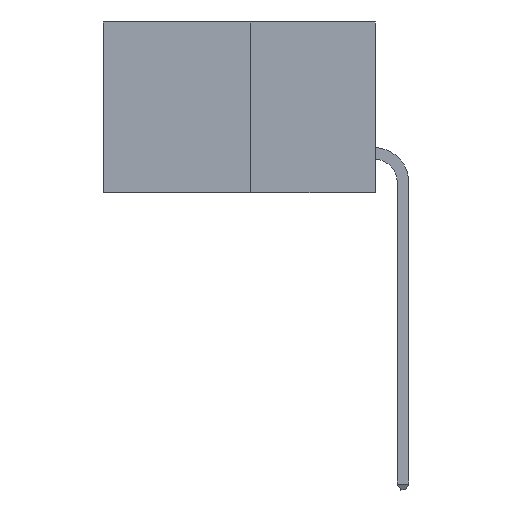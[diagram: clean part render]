
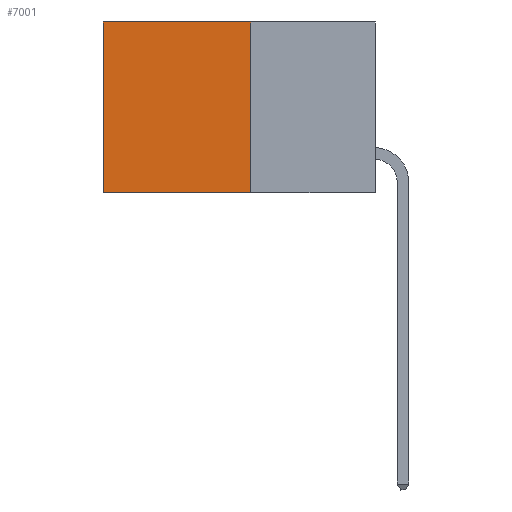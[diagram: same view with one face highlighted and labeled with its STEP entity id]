
A CAD part, left-side view. The second image highlights one B-rep face of the part: STEP entity #7001.
In plain terms, the highlighted planar face has unit normal (-1, 0, 0).
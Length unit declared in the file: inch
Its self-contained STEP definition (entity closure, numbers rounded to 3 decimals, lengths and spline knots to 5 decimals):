
#59 = CARTESIAN_POINT ( 'NONE',  ( 0.277, 0.27, -0.37 ) ) ;
#160 = DIRECTION ( 'NONE',  ( 0., 1., 0. ) ) ;
#420 = VECTOR ( 'NONE', #11114, 39.37008 ) ;
#424 = ORIENTED_EDGE ( 'NONE', *, *, #3359, .T. ) ;
#548 = ORIENTED_EDGE ( 'NONE', *, *, #3813, .T. ) ;
#681 = FACE_OUTER_BOUND ( 'NONE', #6501, .T. ) ;
#788 = LINE ( 'NONE', #7457, #10775 ) ;
#984 = DIRECTION ( 'NONE',  ( 0., 0., -1. ) ) ;
#1108 = LINE ( 'NONE', #9748, #420 ) ;
#2224 = CARTESIAN_POINT ( 'NONE',  ( 0.277, 0.59, -0.37 ) ) ;
#2592 = DIRECTION ( 'NONE',  ( 0., 0., -1. ) ) ;
#3055 = ORIENTED_EDGE ( 'NONE', *, *, #3222, .F. ) ;
#3222 = EDGE_CURVE ( 'NONE', #3779, #10285, #10219, .T. ) ;
#3359 = EDGE_CURVE ( 'NONE', #5537, #12419, #10066, .T. ) ;
#3399 = ORIENTED_EDGE ( 'NONE', *, *, #9076, .F. ) ;
#3779 = VERTEX_POINT ( 'NONE', #4586 ) ;
#3813 = EDGE_CURVE ( 'NONE', #12419, #10285, #1108, .T. ) ;
#4586 = CARTESIAN_POINT ( 'NONE',  ( 0.277, 0.27, -0.37 ) ) ;
#4890 = CARTESIAN_POINT ( 'NONE',  ( 0.277, 0.27, 0. ) ) ;
#5537 = VERTEX_POINT ( 'NONE', #4890 ) ;
#6043 = AXIS2_PLACEMENT_3D ( 'NONE', #12412, #7006, #984 ) ;
#6501 = EDGE_LOOP ( 'NONE', ( #548, #3055, #3399, #424 ) ) ;
#6963 = PLANE ( 'NONE',  #6043 ) ;
#7001 = ADVANCED_FACE ( 'NONE', ( #681 ), #6963, .F. ) ;
#7006 = DIRECTION ( 'NONE',  ( 1., 0., 0. ) ) ;
#7457 = CARTESIAN_POINT ( 'NONE',  ( 0.277, 0.27, -0.37 ) ) ;
#7536 = VECTOR ( 'NONE', #160, 39.37008 ) ;
#8968 = DIRECTION ( 'NONE',  ( 0., 1., 0. ) ) ;
#9076 = EDGE_CURVE ( 'NONE', #5537, #3779, #788, .T. ) ;
#9748 = CARTESIAN_POINT ( 'NONE',  ( 0.277, 0.59, -0.37 ) ) ;
#10066 = LINE ( 'NONE', #11201, #12186 ) ;
#10219 = LINE ( 'NONE', #59, #7536 ) ;
#10285 = VERTEX_POINT ( 'NONE', #2224 ) ;
#10775 = VECTOR ( 'NONE', #2592, 39.37008 ) ;
#11114 = DIRECTION ( 'NONE',  ( 0., 0., -1. ) ) ;
#11201 = CARTESIAN_POINT ( 'NONE',  ( 0.277, 0.27, 0. ) ) ;
#12186 = VECTOR ( 'NONE', #8968, 39.37008 ) ;
#12346 = CARTESIAN_POINT ( 'NONE',  ( 0.277, 0.59, 0. ) ) ;
#12412 = CARTESIAN_POINT ( 'NONE',  ( 0.277, 0.27, -0.37 ) ) ;
#12419 = VERTEX_POINT ( 'NONE', #12346 ) ;
